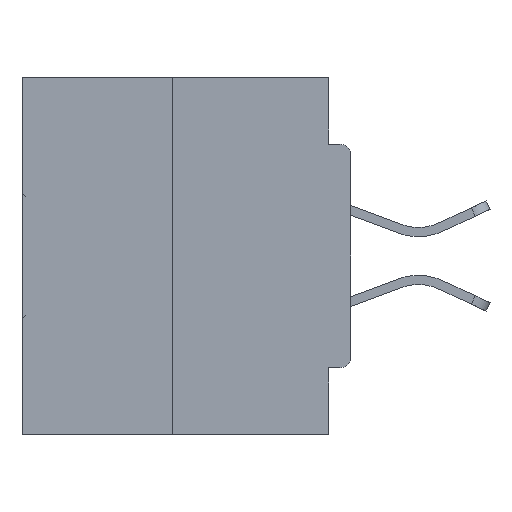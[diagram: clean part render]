
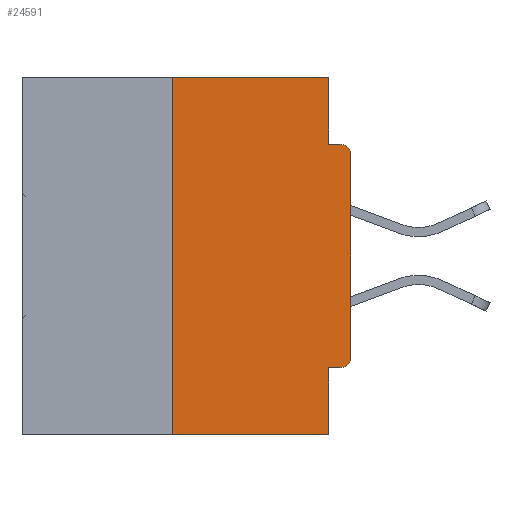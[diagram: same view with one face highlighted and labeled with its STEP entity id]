
A CAD part, left-side view. The second image highlights one B-rep face of the part: STEP entity #24591.
In plain terms, the highlighted planar face has unit normal (-1, 0, 0).
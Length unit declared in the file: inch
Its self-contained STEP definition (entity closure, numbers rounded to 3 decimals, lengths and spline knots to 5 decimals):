
#26 = VERTEX_POINT ( 'NONE', #14741 ) ;
#224 = VECTOR ( 'NONE', #18344, 39.37008 ) ;
#706 = CARTESIAN_POINT ( 'NONE',  ( 0., 0., -0.0935 ) ) ;
#1109 = CARTESIAN_POINT ( 'NONE',  ( 0., 0.46, 0. ) ) ;
#1298 = CARTESIAN_POINT ( 'NONE',  ( 0., 0., 0. ) ) ;
#1350 = VERTEX_POINT ( 'NONE', #28045 ) ;
#2079 = DIRECTION ( 'NONE',  ( 0., 0., -1. ) ) ;
#2139 = CARTESIAN_POINT ( 'NONE',  ( 0., 0., -0.1085 ) ) ;
#2941 = AXIS2_PLACEMENT_3D ( 'NONE', #1109, #17926, #40539 ) ;
#3280 = EDGE_CURVE ( 'NONE', #17690, #1350, #42604, .T. ) ;
#4082 = CARTESIAN_POINT ( 'NONE',  ( 0., 0.46, -0.5 ) ) ;
#4759 = ORIENTED_EDGE ( 'NONE', *, *, #33029, .F. ) ;
#5815 = VECTOR ( 'NONE', #14066, 39.37008 ) ;
#6768 = LINE ( 'NONE', #4082, #33160 ) ;
#7142 = DIRECTION ( 'NONE',  ( -1., 0., 0. ) ) ;
#7460 = LINE ( 'NONE', #17649, #33304 ) ;
#7563 = VERTEX_POINT ( 'NONE', #31290 ) ;
#7624 = PLANE ( 'NONE',  #2941 ) ;
#8120 = DIRECTION ( 'NONE',  ( 0., -1., 0. ) ) ;
#9725 = ORIENTED_EDGE ( 'NONE', *, *, #33473, .F. ) ;
#9941 = CARTESIAN_POINT ( 'NONE',  ( 0., 0.031, -0.4065 ) ) ;
#10948 = VERTEX_POINT ( 'NONE', #2139 ) ;
#12470 = ORIENTED_EDGE ( 'NONE', *, *, #39909, .F. ) ;
#13530 = DIRECTION ( 'NONE',  ( 0., 0., -1. ) ) ;
#14066 = DIRECTION ( 'NONE',  ( 0., -1., 0. ) ) ;
#14121 = LINE ( 'NONE', #706, #5815 ) ;
#14364 = DIRECTION ( 'NONE',  ( 0., 0., -1. ) ) ;
#14741 = CARTESIAN_POINT ( 'NONE',  ( 0., 0.031, 0. ) ) ;
#14955 = EDGE_CURVE ( 'NONE', #17749, #37122, #33495, .T. ) ;
#15068 = AXIS2_PLACEMENT_3D ( 'NONE', #30091, #7142, #13530 ) ;
#15115 = CARTESIAN_POINT ( 'NONE',  ( 0., 0., -0.3915 ) ) ;
#15459 = EDGE_CURVE ( 'NONE', #10948, #32432, #42164, .T. ) ;
#16332 = ORIENTED_EDGE ( 'NONE', *, *, #29214, .T. ) ;
#16338 = LINE ( 'NONE', #39675, #32862 ) ;
#16343 = LINE ( 'NONE', #38328, #30783 ) ;
#17649 = CARTESIAN_POINT ( 'NONE',  ( 0., 0.031, 0. ) ) ;
#17654 = ORIENTED_EDGE ( 'NONE', *, *, #15459, .T. ) ;
#17690 = VERTEX_POINT ( 'NONE', #19939 ) ;
#17749 = VERTEX_POINT ( 'NONE', #9941 ) ;
#17926 = DIRECTION ( 'NONE',  ( 1., 0., 0. ) ) ;
#18022 = DIRECTION ( 'NONE',  ( -1., 0., 0. ) ) ;
#18258 = ORIENTED_EDGE ( 'NONE', *, *, #14955, .F. ) ;
#18344 = DIRECTION ( 'NONE',  ( 0., 0., 1. ) ) ;
#18426 = DIRECTION ( 'NONE',  ( 0., 0., -1. ) ) ;
#18488 = CARTESIAN_POINT ( 'NONE',  ( 0., 0.25, 0. ) ) ;
#18536 = EDGE_CURVE ( 'NONE', #7563, #38694, #19264, .T. ) ;
#19264 = CIRCLE ( 'NONE', #15068, 0.015 ) ;
#19398 = CARTESIAN_POINT ( 'NONE',  ( 0., 0.031, -0.0935 ) ) ;
#19570 = VECTOR ( 'NONE', #14364, 39.37008 ) ;
#19939 = CARTESIAN_POINT ( 'NONE',  ( 0., 0.25, -0.5 ) ) ;
#21144 = DIRECTION ( 'NONE',  ( 0., 0., 1. ) ) ;
#21346 = ORIENTED_EDGE ( 'NONE', *, *, #18536, .T. ) ;
#21925 = FACE_OUTER_BOUND ( 'NONE', #30506, .T. ) ;
#23155 = VERTEX_POINT ( 'NONE', #19398 ) ;
#23575 = EDGE_CURVE ( 'NONE', #1350, #26, #16343, .T. ) ;
#23986 = ORIENTED_EDGE ( 'NONE', *, *, #40562, .T. ) ;
#24591 = ADVANCED_FACE ( 'NONE', ( #21925 ), #7624, .F. ) ;
#26798 = CARTESIAN_POINT ( 'NONE',  ( 0., 0.015, -0.0935 ) ) ;
#28045 = CARTESIAN_POINT ( 'NONE',  ( 0., 0.25, 0. ) ) ;
#29078 = LINE ( 'NONE', #1298, #30642 ) ;
#29214 = EDGE_CURVE ( 'NONE', #38694, #10948, #29078, .T. ) ;
#30091 = CARTESIAN_POINT ( 'NONE',  ( 0., 0.015, -0.3915 ) ) ;
#30506 = EDGE_LOOP ( 'NONE', ( #32926, #39296, #23986, #18258, #4759, #21346, #16332, #17654, #12470, #9725 ) ) ;
#30642 = VECTOR ( 'NONE', #21144, 39.37008 ) ;
#30783 = VECTOR ( 'NONE', #8120, 39.37008 ) ;
#30940 = CARTESIAN_POINT ( 'NONE',  ( 0., 0.031, -0.5 ) ) ;
#31290 = CARTESIAN_POINT ( 'NONE',  ( 0., 0.015, -0.4065 ) ) ;
#32432 = VERTEX_POINT ( 'NONE', #26798 ) ;
#32862 = VECTOR ( 'NONE', #32945, 39.37008 ) ;
#32926 = ORIENTED_EDGE ( 'NONE', *, *, #23575, .F. ) ;
#32945 = DIRECTION ( 'NONE',  ( 0., 1., 0. ) ) ;
#33029 = EDGE_CURVE ( 'NONE', #7563, #17749, #16338, .T. ) ;
#33160 = VECTOR ( 'NONE', #40073, 39.37008 ) ;
#33304 = VECTOR ( 'NONE', #2079, 39.37008 ) ;
#33473 = EDGE_CURVE ( 'NONE', #26, #23155, #7460, .T. ) ;
#33495 = LINE ( 'NONE', #30940, #19570 ) ;
#37122 = VERTEX_POINT ( 'NONE', #38258 ) ;
#37765 = CARTESIAN_POINT ( 'NONE',  ( 0., 0.015, -0.1085 ) ) ;
#38258 = CARTESIAN_POINT ( 'NONE',  ( 0., 0.031, -0.5 ) ) ;
#38328 = CARTESIAN_POINT ( 'NONE',  ( 0., 0.46, 0. ) ) ;
#38694 = VERTEX_POINT ( 'NONE', #15115 ) ;
#39296 = ORIENTED_EDGE ( 'NONE', *, *, #3280, .F. ) ;
#39675 = CARTESIAN_POINT ( 'NONE',  ( 0., 0., -0.4065 ) ) ;
#39909 = EDGE_CURVE ( 'NONE', #23155, #32432, #14121, .T. ) ;
#40073 = DIRECTION ( 'NONE',  ( 0., -1., 0. ) ) ;
#40539 = DIRECTION ( 'NONE',  ( 0., 0., -1. ) ) ;
#40562 = EDGE_CURVE ( 'NONE', #17690, #37122, #6768, .T. ) ;
#41193 = AXIS2_PLACEMENT_3D ( 'NONE', #37765, #18022, #18426 ) ;
#42164 = CIRCLE ( 'NONE', #41193, 0.015 ) ;
#42604 = LINE ( 'NONE', #18488, #224 ) ;
